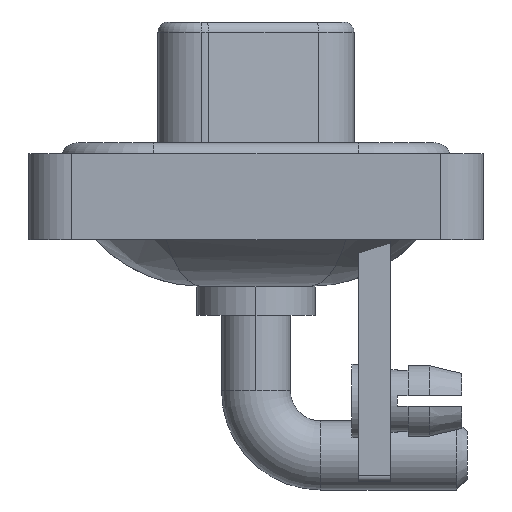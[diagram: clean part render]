
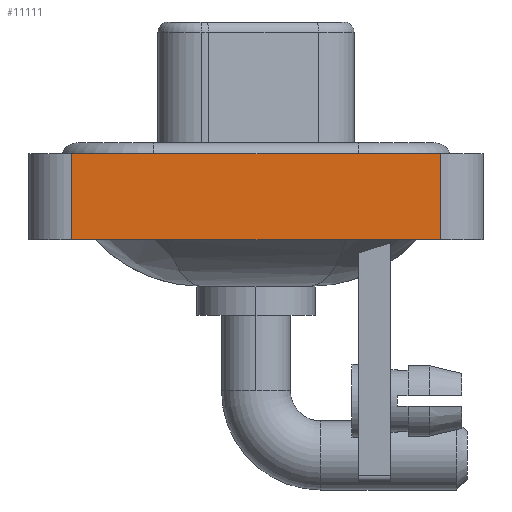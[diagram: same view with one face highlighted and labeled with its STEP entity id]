
A CAD part, left-side view. The second image highlights one B-rep face of the part: STEP entity #11111.
In plain terms, the highlighted planar face has unit normal (-1, 0, 0).
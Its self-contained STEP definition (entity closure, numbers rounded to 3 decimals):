
#281 = ORIENTED_EDGE ( 'NONE', *, *, #11327, .T. ) ;
#708 = VECTOR ( 'NONE', #13714, 1000. ) ;
#1404 = LINE ( 'NONE', #8040, #708 ) ;
#1447 = ORIENTED_EDGE ( 'NONE', *, *, #5815, .T. ) ;
#1497 = ORIENTED_EDGE ( 'NONE', *, *, #9483, .F. ) ;
#1514 = VERTEX_POINT ( 'NONE', #4913 ) ;
#1670 = AXIS2_PLACEMENT_3D ( 'NONE', #6990, #15041, #12664 ) ;
#2139 = CARTESIAN_POINT ( 'NONE',  ( -7.25, 8.55, -3.6 ) ) ;
#2752 = LINE ( 'NONE', #13463, #15345 ) ;
#4133 = CARTESIAN_POINT ( 'NONE',  ( -7.25, 8.55, -3.6 ) ) ;
#4913 = CARTESIAN_POINT ( 'NONE',  ( -7.25, -8.55, 0.4 ) ) ;
#5815 = EDGE_CURVE ( 'NONE', #13694, #13516, #1404, .T. ) ;
#6990 = CARTESIAN_POINT ( 'NONE',  ( -7.25, -8.55, -3.6 ) ) ;
#7167 = FACE_OUTER_BOUND ( 'NONE', #13836, .T. ) ;
#7894 = DIRECTION ( 'NONE',  ( 0., -1., 0. ) ) ;
#7955 = LINE ( 'NONE', #10899, #11002 ) ;
#8040 = CARTESIAN_POINT ( 'NONE',  ( -7.25, -8.55, -3.6 ) ) ;
#8367 = DIRECTION ( 'NONE',  ( 0., 0., 1. ) ) ;
#8733 = VECTOR ( 'NONE', #8367, 1000. ) ;
#8786 = VERTEX_POINT ( 'NONE', #11866 ) ;
#9483 = EDGE_CURVE ( 'NONE', #8786, #1514, #2752, .T. ) ;
#10319 = CARTESIAN_POINT ( 'NONE',  ( -7.25, -8.55, -3.6 ) ) ;
#10899 = CARTESIAN_POINT ( 'NONE',  ( -7.25, -8.55, -3.6 ) ) ;
#11002 = VECTOR ( 'NONE', #11873, 1000. ) ;
#11089 = PLANE ( 'NONE',  #1670 ) ;
#11111 = ADVANCED_FACE ( 'NONE', ( #7167 ), #11089, .T. ) ;
#11226 = ORIENTED_EDGE ( 'NONE', *, *, #12023, .F. ) ;
#11327 = EDGE_CURVE ( 'NONE', #13516, #1514, #7955, .T. ) ;
#11866 = CARTESIAN_POINT ( 'NONE',  ( -7.25, 8.55, 0.4 ) ) ;
#11873 = DIRECTION ( 'NONE',  ( 0., 0., 1. ) ) ;
#12023 = EDGE_CURVE ( 'NONE', #13694, #8786, #16394, .T. ) ;
#12664 = DIRECTION ( 'NONE',  ( 0., 0., 1. ) ) ;
#13463 = CARTESIAN_POINT ( 'NONE',  ( -7.25, -8.55, 0.4 ) ) ;
#13516 = VERTEX_POINT ( 'NONE', #10319 ) ;
#13694 = VERTEX_POINT ( 'NONE', #2139 ) ;
#13714 = DIRECTION ( 'NONE',  ( 0., -1., 0. ) ) ;
#13836 = EDGE_LOOP ( 'NONE', ( #281, #1497, #11226, #1447 ) ) ;
#15041 = DIRECTION ( 'NONE',  ( -1., 0., 0. ) ) ;
#15345 = VECTOR ( 'NONE', #7894, 1000. ) ;
#16394 = LINE ( 'NONE', #4133, #8733 ) ;
